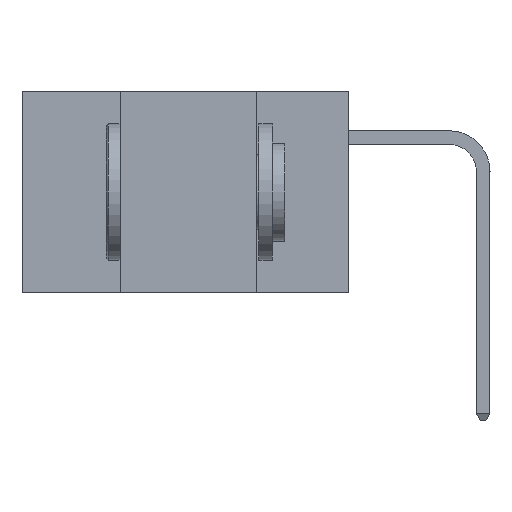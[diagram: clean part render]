
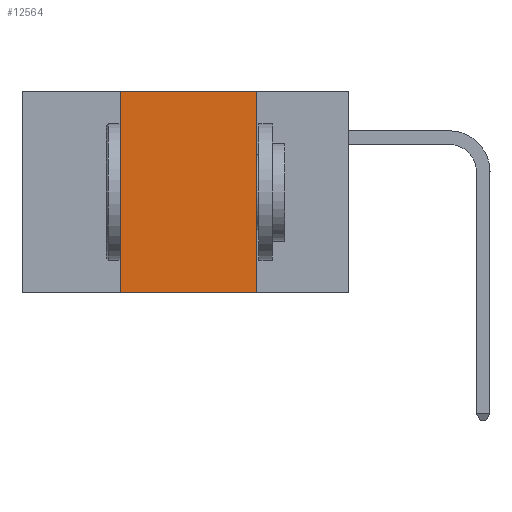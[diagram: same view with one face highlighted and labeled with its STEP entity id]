
A CAD part, left-side view. The second image highlights one B-rep face of the part: STEP entity #12564.
In plain terms, the highlighted planar face has unit normal (-1, 0, 0).
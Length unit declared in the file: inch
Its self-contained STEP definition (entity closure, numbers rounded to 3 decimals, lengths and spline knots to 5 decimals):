
#489 = ORIENTED_EDGE ( 'NONE', *, *, #19008, .T. ) ;
#1362 = CARTESIAN_POINT ( 'NONE',  ( 0., 0.17, 0. ) ) ;
#1381 = CARTESIAN_POINT ( 'NONE',  ( 0., 0.6, -0.37 ) ) ;
#1552 = CARTESIAN_POINT ( 'NONE',  ( 0., 0.6, 0. ) ) ;
#3017 = LINE ( 'NONE', #7308, #17476 ) ;
#4675 = VERTEX_POINT ( 'NONE', #10348 ) ;
#5008 = CARTESIAN_POINT ( 'NONE',  ( 0., 0.42, -0.37 ) ) ;
#5883 = DIRECTION ( 'NONE',  ( 0., -1., 0. ) ) ;
#7308 = CARTESIAN_POINT ( 'NONE',  ( 0., 0.42, 0. ) ) ;
#7390 = PLANE ( 'NONE',  #32374 ) ;
#10141 = DIRECTION ( 'NONE',  ( 0., 0., -1. ) ) ;
#10158 = DIRECTION ( 'NONE',  ( 0., -1., 0. ) ) ;
#10338 = DIRECTION ( 'NONE',  ( 0., 0., -1. ) ) ;
#10348 = CARTESIAN_POINT ( 'NONE',  ( 0., 0.42, 0. ) ) ;
#12564 = ADVANCED_FACE ( 'NONE', ( #36441 ), #7390, .F. ) ;
#14045 = VECTOR ( 'NONE', #10158, 39.37008 ) ;
#15022 = VECTOR ( 'NONE', #10141, 39.37008 ) ;
#15497 = VERTEX_POINT ( 'NONE', #5008 ) ;
#15605 = ORIENTED_EDGE ( 'NONE', *, *, #28500, .F. ) ;
#17476 = VECTOR ( 'NONE', #27367, 39.37008 ) ;
#17499 = EDGE_CURVE ( 'NONE', #4675, #28470, #21326, .T. ) ;
#17522 = ORIENTED_EDGE ( 'NONE', *, *, #26649, .F. ) ;
#19008 = EDGE_CURVE ( 'NONE', #15497, #27258, #21663, .T. ) ;
#19547 = VECTOR ( 'NONE', #5883, 39.37008 ) ;
#21326 = LINE ( 'NONE', #34352, #19547 ) ;
#21663 = LINE ( 'NONE', #1381, #14045 ) ;
#22672 = LINE ( 'NONE', #1362, #15022 ) ;
#24341 = CARTESIAN_POINT ( 'NONE',  ( 0., 0.17, -0.37 ) ) ;
#26629 = ORIENTED_EDGE ( 'NONE', *, *, #17499, .F. ) ;
#26649 = EDGE_CURVE ( 'NONE', #15497, #4675, #3017, .T. ) ;
#27258 = VERTEX_POINT ( 'NONE', #24341 ) ;
#27367 = DIRECTION ( 'NONE',  ( 0., 0., 1. ) ) ;
#27446 = DIRECTION ( 'NONE',  ( 1., 0., 0. ) ) ;
#28470 = VERTEX_POINT ( 'NONE', #29947 ) ;
#28500 = EDGE_CURVE ( 'NONE', #28470, #27258, #22672, .T. ) ;
#29947 = CARTESIAN_POINT ( 'NONE',  ( 0., 0.17, 0. ) ) ;
#32374 = AXIS2_PLACEMENT_3D ( 'NONE', #1552, #27446, #10338 ) ;
#34352 = CARTESIAN_POINT ( 'NONE',  ( 0., 0.6, 0. ) ) ;
#34777 = EDGE_LOOP ( 'NONE', ( #15605, #26629, #17522, #489 ) ) ;
#36441 = FACE_OUTER_BOUND ( 'NONE', #34777, .T. ) ;
